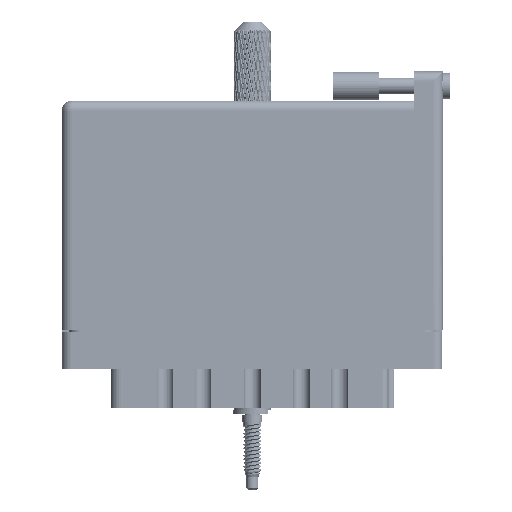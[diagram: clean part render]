
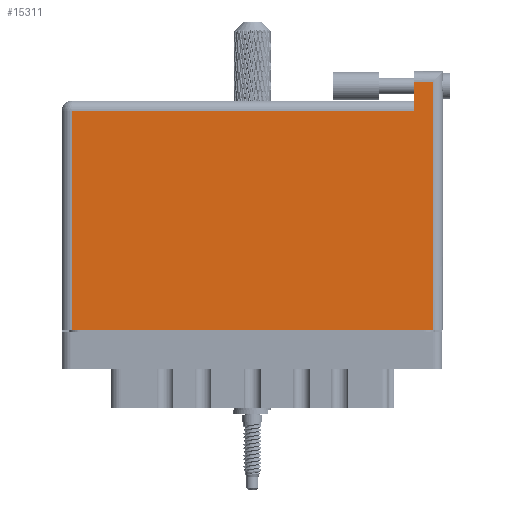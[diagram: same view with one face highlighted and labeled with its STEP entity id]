
A CAD part, front view. The second image highlights one B-rep face of the part: STEP entity #15311.
In plain terms, the highlighted face is planar.
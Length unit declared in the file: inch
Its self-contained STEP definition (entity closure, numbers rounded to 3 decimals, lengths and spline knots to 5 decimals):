
#7575 = CARTESIAN_POINT ( 'NONE',  ( 2.53, 0., 0. ) ) ;
#9828 = DIRECTION ( 'NONE',  ( 0., 1., 0. ) ) ;
#10827 = CARTESIAN_POINT ( 'NONE',  ( 0., 1.696, 0. ) ) ;
#15311 = ADVANCED_FACE ( 'NONE', ( #94067 ), #48952, .F. ) ;
#16291 = VECTOR ( 'NONE', #63875, 39.37008 ) ;
#18448 = VERTEX_POINT ( 'NONE', #97674 ) ;
#31388 = EDGE_CURVE ( 'NONE', #18448, #73883, #78190, .T. ) ;
#31597 = EDGE_CURVE ( 'NONE', #45149, #54581, #75218, .T. ) ;
#34952 = LINE ( 'NONE', #109680, #16291 ) ;
#35230 = CARTESIAN_POINT ( 'NONE',  ( 2.53, 1.696, 0. ) ) ;
#35631 = DIRECTION ( 'NONE',  ( 1., 0., 0. ) ) ;
#37184 = VERTEX_POINT ( 'NONE', #7575 ) ;
#40489 = DIRECTION ( 'NONE',  ( 0., -1., 0. ) ) ;
#41184 = EDGE_LOOP ( 'NONE', ( #61953, #62066, #97781, #69102, #102373, #65857 ) ) ;
#45149 = VERTEX_POINT ( 'NONE', #35230 ) ;
#45682 = VECTOR ( 'NONE', #35631, 39.37008 ) ;
#47196 = EDGE_CURVE ( 'NONE', #37184, #45149, #101691, .T. ) ;
#48494 = CARTESIAN_POINT ( 'NONE',  ( 2.403, 1.696, 0. ) ) ;
#48952 = PLANE ( 'NONE',  #82286 ) ;
#49381 = VECTOR ( 'NONE', #107725, 39.37008 ) ;
#51638 = VERTEX_POINT ( 'NONE', #112546 ) ;
#54581 = VERTEX_POINT ( 'NONE', #48494 ) ;
#55894 = LINE ( 'NONE', #113618, #65897 ) ;
#58164 = DIRECTION ( 'NONE',  ( -1., 0., 0. ) ) ;
#61953 = ORIENTED_EDGE ( 'NONE', *, *, #78360, .T. ) ;
#62066 = ORIENTED_EDGE ( 'NONE', *, *, #47196, .T. ) ;
#62797 = VECTOR ( 'NONE', #9828, 39.37008 ) ;
#63875 = DIRECTION ( 'NONE',  ( -1., 0., 0. ) ) ;
#65110 = CARTESIAN_POINT ( 'NONE',  ( 0.07, 0., 0. ) ) ;
#65857 = ORIENTED_EDGE ( 'NONE', *, *, #31388, .T. ) ;
#65897 = VECTOR ( 'NONE', #40489, 39.37008 ) ;
#68621 = LINE ( 'NONE', #73372, #45682 ) ;
#69102 = ORIENTED_EDGE ( 'NONE', *, *, #101376, .T. ) ;
#69422 = VECTOR ( 'NONE', #85210, 39.37008 ) ;
#73348 = CARTESIAN_POINT ( 'NONE',  ( 2.53, 1.766, 0. ) ) ;
#73372 = CARTESIAN_POINT ( 'NONE',  ( 0., 0., 0. ) ) ;
#73883 = VERTEX_POINT ( 'NONE', #65110 ) ;
#75218 = LINE ( 'NONE', #10827, #69422 ) ;
#78190 = LINE ( 'NONE', #90903, #49381 ) ;
#78360 = EDGE_CURVE ( 'NONE', #73883, #37184, #68621, .T. ) ;
#82286 = AXIS2_PLACEMENT_3D ( 'NONE', #103985, #113224, #58164 ) ;
#85210 = DIRECTION ( 'NONE',  ( -1., 0., 0. ) ) ;
#90903 = CARTESIAN_POINT ( 'NONE',  ( 0.07, 0., 0. ) ) ;
#94067 = FACE_OUTER_BOUND ( 'NONE', #41184, .T. ) ;
#97674 = CARTESIAN_POINT ( 'NONE',  ( 0.07, 1.496, 0. ) ) ;
#97781 = ORIENTED_EDGE ( 'NONE', *, *, #31597, .T. ) ;
#101376 = EDGE_CURVE ( 'NONE', #54581, #51638, #55894, .T. ) ;
#101691 = LINE ( 'NONE', #73348, #62797 ) ;
#102373 = ORIENTED_EDGE ( 'NONE', *, *, #109752, .T. ) ;
#103985 = CARTESIAN_POINT ( 'NONE',  ( 0., 1.566, 0. ) ) ;
#107725 = DIRECTION ( 'NONE',  ( 0., -1., 0. ) ) ;
#109680 = CARTESIAN_POINT ( 'NONE',  ( 0., 1.496, 0. ) ) ;
#109752 = EDGE_CURVE ( 'NONE', #51638, #18448, #34952, .T. ) ;
#112546 = CARTESIAN_POINT ( 'NONE',  ( 2.403, 1.496, 0. ) ) ;
#113224 = DIRECTION ( 'NONE',  ( 0., 0., -1. ) ) ;
#113618 = CARTESIAN_POINT ( 'NONE',  ( 2.403, 1.766, 0. ) ) ;
